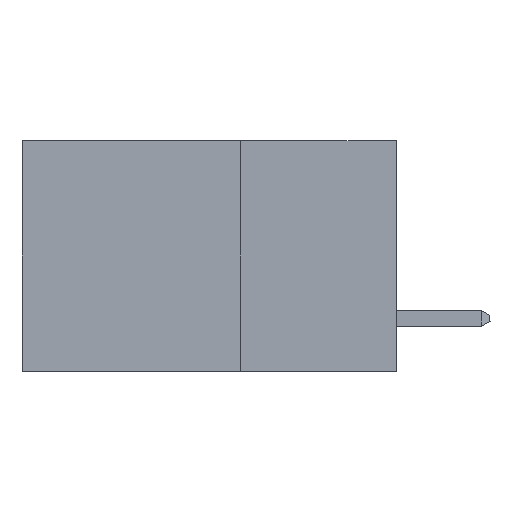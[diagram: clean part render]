
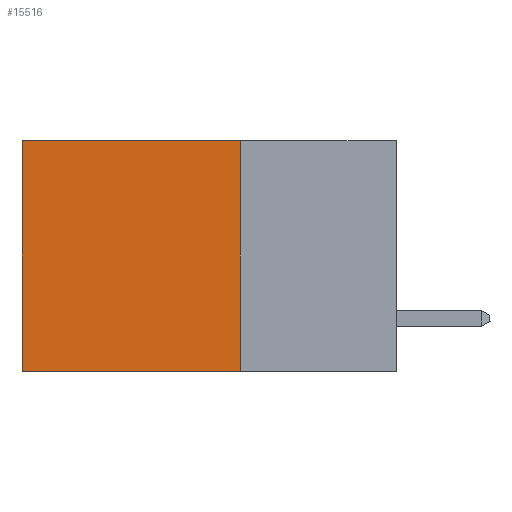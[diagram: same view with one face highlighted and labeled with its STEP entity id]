
A CAD part, left-side view. The second image highlights one B-rep face of the part: STEP entity #15516.
In plain terms, the highlighted planar face has unit normal (-1, 0, 0).
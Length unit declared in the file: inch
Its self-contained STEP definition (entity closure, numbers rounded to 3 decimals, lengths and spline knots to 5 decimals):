
#278 = VERTEX_POINT ( 'NONE', #15155 ) ;
#291 = VERTEX_POINT ( 'NONE', #2202 ) ;
#588 = LINE ( 'NONE', #15039, #9799 ) ;
#927 = CARTESIAN_POINT ( 'NONE',  ( 0.298, 0.6, 0. ) ) ;
#1038 = DIRECTION ( 'NONE',  ( 1., 0., 0. ) ) ;
#1218 = EDGE_CURVE ( 'NONE', #11356, #1679, #588, .T. ) ;
#1679 = VERTEX_POINT ( 'NONE', #7951 ) ;
#2202 = CARTESIAN_POINT ( 'NONE',  ( 0.298, 0.6, 0. ) ) ;
#2525 = CARTESIAN_POINT ( 'NONE',  ( 0.298, 0.25, 0. ) ) ;
#3901 = LINE ( 'NONE', #2525, #6835 ) ;
#4059 = FACE_OUTER_BOUND ( 'NONE', #12633, .T. ) ;
#6312 = DIRECTION ( 'NONE',  ( 0., 1., 0. ) ) ;
#6786 = DIRECTION ( 'NONE',  ( 0., 1., 0. ) ) ;
#6835 = VECTOR ( 'NONE', #6312, 39.37008 ) ;
#7951 = CARTESIAN_POINT ( 'NONE',  ( 0.298, 0.25, -0.37 ) ) ;
#8027 = ORIENTED_EDGE ( 'NONE', *, *, #10757, .T. ) ;
#8316 = CARTESIAN_POINT ( 'NONE',  ( 0.298, 0.25, 0. ) ) ;
#8551 = PLANE ( 'NONE',  #10536 ) ;
#8986 = DIRECTION ( 'NONE',  ( 0., 0., -1. ) ) ;
#9194 = CARTESIAN_POINT ( 'NONE',  ( 0.298, 0.25, -0.37 ) ) ;
#9774 = DIRECTION ( 'NONE',  ( 0., 0., -1. ) ) ;
#9799 = VECTOR ( 'NONE', #8986, 39.37008 ) ;
#10536 = AXIS2_PLACEMENT_3D ( 'NONE', #12101, #1038, #9774 ) ;
#10757 = EDGE_CURVE ( 'NONE', #291, #278, #14367, .T. ) ;
#10827 = VECTOR ( 'NONE', #10844, 39.37008 ) ;
#10844 = DIRECTION ( 'NONE',  ( 0., 0., -1. ) ) ;
#11225 = ORIENTED_EDGE ( 'NONE', *, *, #12560, .F. ) ;
#11356 = VERTEX_POINT ( 'NONE', #8316 ) ;
#11617 = ORIENTED_EDGE ( 'NONE', *, *, #14996, .T. ) ;
#11999 = VECTOR ( 'NONE', #6786, 39.37008 ) ;
#12101 = CARTESIAN_POINT ( 'NONE',  ( 0.298, 0.25, 0. ) ) ;
#12360 = LINE ( 'NONE', #9194, #11999 ) ;
#12560 = EDGE_CURVE ( 'NONE', #1679, #278, #12360, .T. ) ;
#12633 = EDGE_LOOP ( 'NONE', ( #8027, #11225, #15529, #11617 ) ) ;
#14367 = LINE ( 'NONE', #927, #10827 ) ;
#14996 = EDGE_CURVE ( 'NONE', #11356, #291, #3901, .T. ) ;
#15039 = CARTESIAN_POINT ( 'NONE',  ( 0.298, 0.25, 0. ) ) ;
#15155 = CARTESIAN_POINT ( 'NONE',  ( 0.298, 0.6, -0.37 ) ) ;
#15516 = ADVANCED_FACE ( 'NONE', ( #4059 ), #8551, .F. ) ;
#15529 = ORIENTED_EDGE ( 'NONE', *, *, #1218, .F. ) ;
